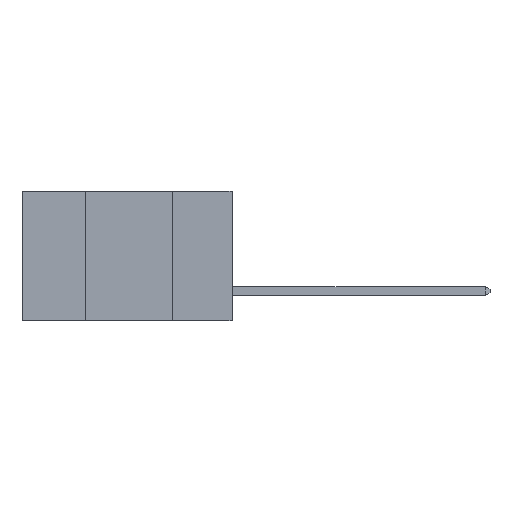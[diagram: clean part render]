
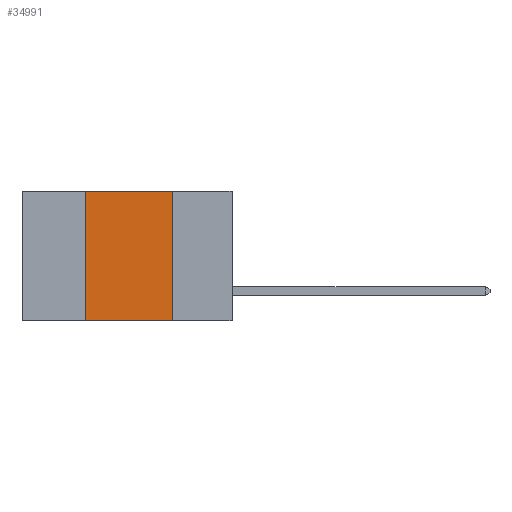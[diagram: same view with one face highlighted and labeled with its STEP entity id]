
A CAD part, left-side view. The second image highlights one B-rep face of the part: STEP entity #34991.
In plain terms, the highlighted planar face has unit normal (-1, 0, 0).
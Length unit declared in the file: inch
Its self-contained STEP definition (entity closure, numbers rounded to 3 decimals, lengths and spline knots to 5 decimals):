
#1001 = EDGE_CURVE ( 'NONE', #25837, #2671, #32454, .T. ) ;
#2048 = CARTESIAN_POINT ( 'NONE',  ( 0., 0.42, -0.37 ) ) ;
#2132 = DIRECTION ( 'NONE',  ( 0., 0., -1. ) ) ;
#2671 = VERTEX_POINT ( 'NONE', #16178 ) ;
#5571 = CARTESIAN_POINT ( 'NONE',  ( 0., 0.42, 0. ) ) ;
#7181 = DIRECTION ( 'NONE',  ( 0., -1., 0. ) ) ;
#8472 = VECTOR ( 'NONE', #21439, 39.37008 ) ;
#9840 = FACE_OUTER_BOUND ( 'NONE', #31987, .T. ) ;
#15758 = ORIENTED_EDGE ( 'NONE', *, *, #17465, .F. ) ;
#16178 = CARTESIAN_POINT ( 'NONE',  ( 0., 0.17, -0.37 ) ) ;
#16634 = CARTESIAN_POINT ( 'NONE',  ( 0., 0.17, 0. ) ) ;
#17465 = EDGE_CURVE ( 'NONE', #20235, #17816, #31435, .T. ) ;
#17586 = LINE ( 'NONE', #16634, #34139 ) ;
#17816 = VERTEX_POINT ( 'NONE', #30856 ) ;
#20235 = VERTEX_POINT ( 'NONE', #5571 ) ;
#20782 = LINE ( 'NONE', #37019, #36325 ) ;
#21157 = DIRECTION ( 'NONE',  ( 1., 0., 0. ) ) ;
#21439 = DIRECTION ( 'NONE',  ( 0., -1., 0. ) ) ;
#21490 = CARTESIAN_POINT ( 'NONE',  ( 0., 0.6, -0.37 ) ) ;
#23101 = EDGE_CURVE ( 'NONE', #17816, #2671, #17586, .T. ) ;
#24688 = DIRECTION ( 'NONE',  ( 0., 0., 1. ) ) ;
#25837 = VERTEX_POINT ( 'NONE', #2048 ) ;
#26018 = ORIENTED_EDGE ( 'NONE', *, *, #39760, .F. ) ;
#30856 = CARTESIAN_POINT ( 'NONE',  ( 0., 0.17, 0. ) ) ;
#31359 = ORIENTED_EDGE ( 'NONE', *, *, #23101, .F. ) ;
#31435 = LINE ( 'NONE', #38443, #39664 ) ;
#31987 = EDGE_LOOP ( 'NONE', ( #31359, #15758, #26018, #38145 ) ) ;
#32454 = LINE ( 'NONE', #21490, #8472 ) ;
#33506 = PLANE ( 'NONE',  #39712 ) ;
#34139 = VECTOR ( 'NONE', #38399, 39.37008 ) ;
#34991 = ADVANCED_FACE ( 'NONE', ( #9840 ), #33506, .F. ) ;
#36325 = VECTOR ( 'NONE', #24688, 39.37008 ) ;
#37019 = CARTESIAN_POINT ( 'NONE',  ( 0., 0.42, 0. ) ) ;
#38145 = ORIENTED_EDGE ( 'NONE', *, *, #1001, .T. ) ;
#38399 = DIRECTION ( 'NONE',  ( 0., 0., -1. ) ) ;
#38443 = CARTESIAN_POINT ( 'NONE',  ( 0., 0.6, 0. ) ) ;
#39664 = VECTOR ( 'NONE', #7181, 39.37008 ) ;
#39712 = AXIS2_PLACEMENT_3D ( 'NONE', #39755, #21157, #2132 ) ;
#39755 = CARTESIAN_POINT ( 'NONE',  ( 0., 0.6, 0. ) ) ;
#39760 = EDGE_CURVE ( 'NONE', #25837, #20235, #20782, .T. ) ;
